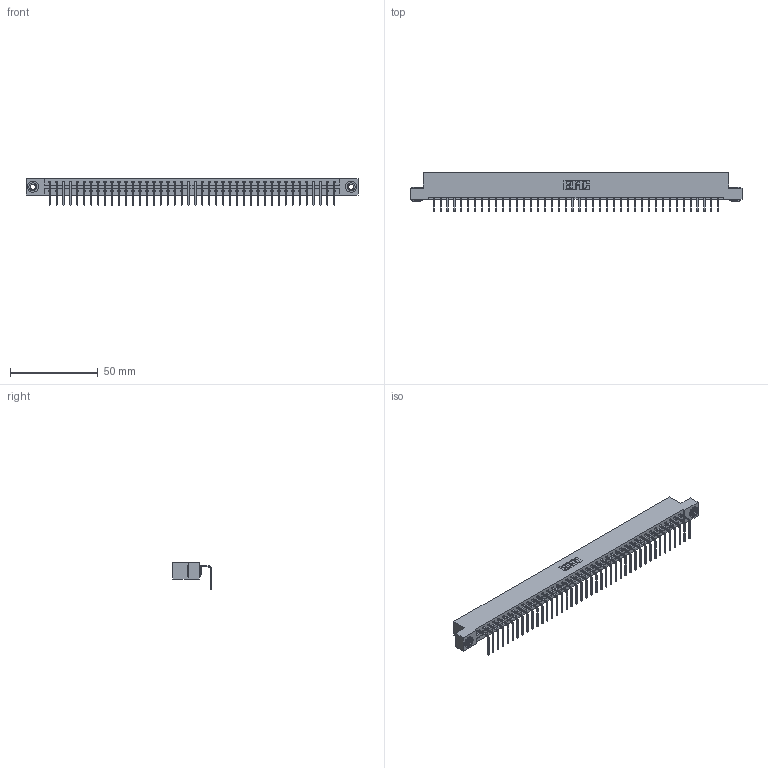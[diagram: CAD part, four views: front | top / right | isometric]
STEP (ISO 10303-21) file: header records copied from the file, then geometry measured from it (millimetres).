
FILE_DESCRIPTION (( 'STEP AP203' ), '1' );
FILE_NAME ('387-042-558-103.STEP', '2018-09-19T23:33:39', ( '' ), ( '' ), 'SwSTEP 2.0', 'SolidWorks 2016', '' );
FILE_SCHEMA (( 'CONFIG_CONTROL_DESIGN' ));
Length unit declared in the file: inch
Products named in the file (4): 345-292-001_558 Tail - 2; 345-250-002_345-250-002-102; 387-042-558-103; 337 Part_Flush Mounting Lugs - 0.156 Dia-TH
Assembly tree (45 placements, depth 2):
  387-042-558-103
    337 Part_Flush Mounting Lugs - 0.156 Dia-TH
    345-292-001_558 Tail - 2  x42
    345-250-002_345-250-002-102  x2
Bounding box: 189.43 x 22.17 x 15.37 mm (x, y, z)
Volume: 19847.7 mm3; surface area: 21602.1 mm2
Topology: 45 solids, 45 shells, 2840 faces, 8535 edges, 5630 vertices
Faces by surface type: plane 2096, cylinder 736, cone 8
Entity records: 31954 total; most frequent: CARTESIAN_POINT 5543, ORIENTED_EDGE 5514, DIRECTION 4699, EDGE_CURVE 2757, VECTOR 2605, LINE 2605, VERTEX_POINT 1834, AXIS2_PLACEMENT_3D 1047
